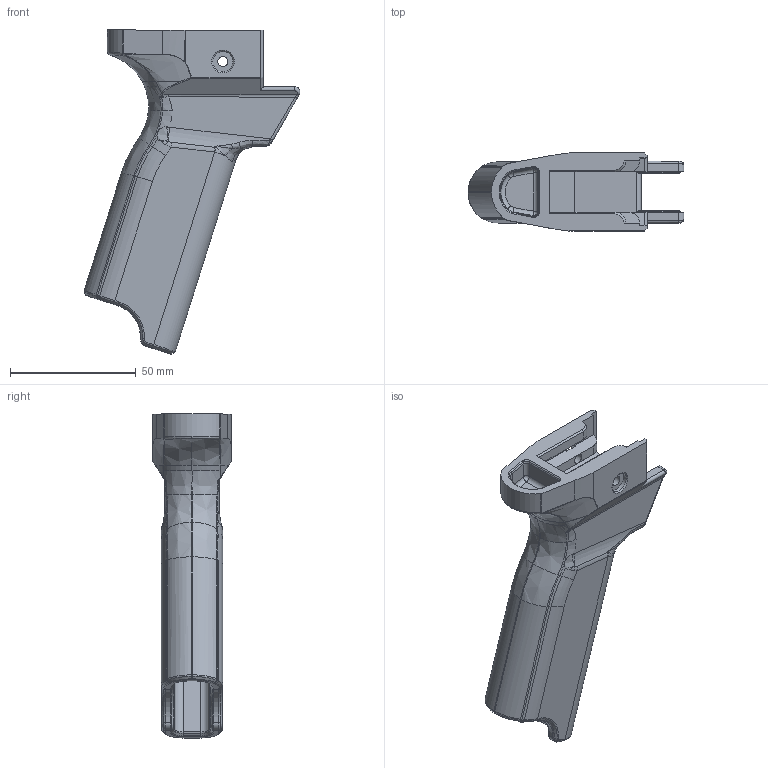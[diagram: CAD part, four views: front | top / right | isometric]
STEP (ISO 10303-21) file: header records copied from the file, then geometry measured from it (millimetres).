
FILE_DESCRIPTION(/* description */ (''),/* implementation_level */ '2;1');
FILE_NAME(/* name */ 'Standard.step',/* time_stamp */ '2021-09-01T03:01:40-04:00',/* author */ (''),/* organization */ (''),/* preprocessor_version */ 'ST-DEVELOPER v18.1',/* originating_system */ 'Autodesk Translation Framework v10.10.0.1391',/* authorisation */ '');
FILE_SCHEMA (('AUTOMOTIVE_DESIGN { 1 0 10303 214 3 1 1 }'));
Length unit declared in the file: millimetre
Products named in the file (1): Standard
Bounding box: 85.78 x 31 x 128.74 mm (x, y, z)
Volume: 72634.1 mm3; surface area: 29099 mm2
Topology: 1 solids, 1 shells, 472 faces, 1146 edges, 655 vertices
Faces by surface type: bspline 143, plane 114, cylinder 103, torus 70, cone 28, sphere 14
Full cylindrical faces by diameter (mm): 4 x2, 8 x1
Entity records: 22512 total; most frequent: CARTESIAN_POINT 12244, ORIENTED_EDGE 2248, DIRECTION 1993, EDGE_CURVE 1124, AXIS2_PLACEMENT_3D 801, VERTEX_POINT 655, EDGE_LOOP 481, FACE_OUTER_BOUND 472
